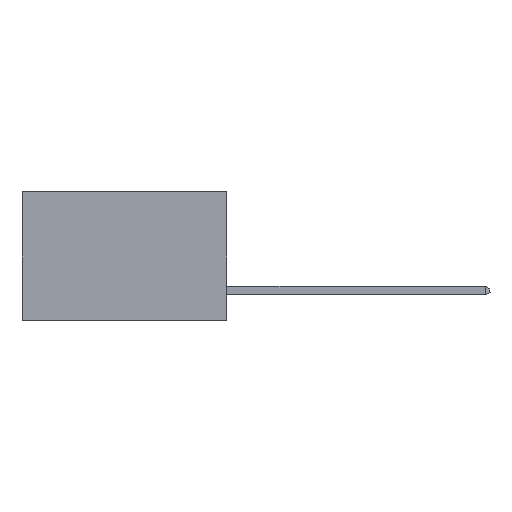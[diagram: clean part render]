
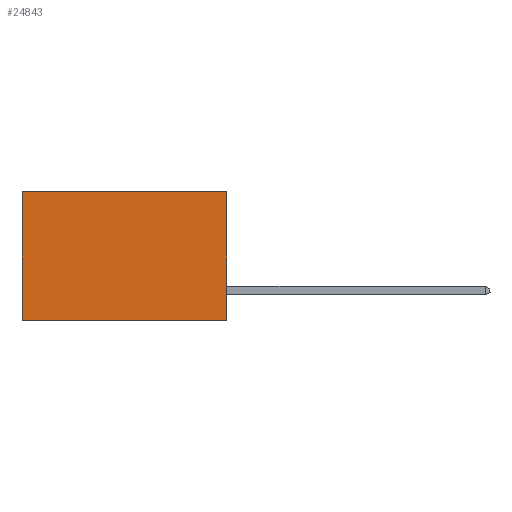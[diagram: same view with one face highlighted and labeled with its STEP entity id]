
A CAD part, left-side view. The second image highlights one B-rep face of the part: STEP entity #24843.
In plain terms, the highlighted planar face has unit normal (-1, 0, 0).
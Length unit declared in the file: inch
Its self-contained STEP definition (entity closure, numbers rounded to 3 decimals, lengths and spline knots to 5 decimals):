
#1145 = CARTESIAN_POINT ( 'NONE',  ( 0.277, 0., -0.37 ) ) ;
#1520 = EDGE_CURVE ( 'NONE', #19059, #19268, #6909, .T. ) ;
#1739 = CARTESIAN_POINT ( 'NONE',  ( 0.277, 0., -0.37 ) ) ;
#2838 = ORIENTED_EDGE ( 'NONE', *, *, #18835, .F. ) ;
#3963 = EDGE_CURVE ( 'NONE', #24043, #19268, #14627, .T. ) ;
#4383 = EDGE_CURVE ( 'NONE', #18365, #24043, #24876, .T. ) ;
#4741 = VECTOR ( 'NONE', #11171, 39.37008 ) ;
#6909 = LINE ( 'NONE', #17982, #11631 ) ;
#7539 = CARTESIAN_POINT ( 'NONE',  ( 0.277, 0., 0. ) ) ;
#7688 = DIRECTION ( 'NONE',  ( 0., 1., 0. ) ) ;
#8595 = PLANE ( 'NONE',  #10168 ) ;
#8858 = ORIENTED_EDGE ( 'NONE', *, *, #4383, .T. ) ;
#9208 = VECTOR ( 'NONE', #7688, 39.37008 ) ;
#10168 = AXIS2_PLACEMENT_3D ( 'NONE', #20492, #10672, #24343 ) ;
#10672 = DIRECTION ( 'NONE',  ( 1., 0., 0. ) ) ;
#11171 = DIRECTION ( 'NONE',  ( 0., 0., -1. ) ) ;
#11631 = VECTOR ( 'NONE', #25083, 39.37008 ) ;
#11786 = EDGE_LOOP ( 'NONE', ( #14855, #16091, #2838, #8858 ) ) ;
#14627 = LINE ( 'NONE', #15504, #24300 ) ;
#14855 = ORIENTED_EDGE ( 'NONE', *, *, #3963, .T. ) ;
#15453 = DIRECTION ( 'NONE',  ( 0., 0., -1. ) ) ;
#15504 = CARTESIAN_POINT ( 'NONE',  ( 0.277, 0.59, -0.37 ) ) ;
#16091 = ORIENTED_EDGE ( 'NONE', *, *, #1520, .F. ) ;
#17982 = CARTESIAN_POINT ( 'NONE',  ( 0.277, 0., -0.37 ) ) ;
#18212 = CARTESIAN_POINT ( 'NONE',  ( 0.277, 0.59, -0.37 ) ) ;
#18365 = VERTEX_POINT ( 'NONE', #19540 ) ;
#18835 = EDGE_CURVE ( 'NONE', #18365, #19059, #20574, .T. ) ;
#19059 = VERTEX_POINT ( 'NONE', #1739 ) ;
#19241 = FACE_OUTER_BOUND ( 'NONE', #11786, .T. ) ;
#19268 = VERTEX_POINT ( 'NONE', #18212 ) ;
#19540 = CARTESIAN_POINT ( 'NONE',  ( 0.277, 0., 0. ) ) ;
#20013 = CARTESIAN_POINT ( 'NONE',  ( 0.277, 0.59, 0. ) ) ;
#20492 = CARTESIAN_POINT ( 'NONE',  ( 0.277, 0., -0.37 ) ) ;
#20574 = LINE ( 'NONE', #1145, #4741 ) ;
#24043 = VERTEX_POINT ( 'NONE', #20013 ) ;
#24300 = VECTOR ( 'NONE', #15453, 39.37008 ) ;
#24343 = DIRECTION ( 'NONE',  ( 0., 0., -1. ) ) ;
#24843 = ADVANCED_FACE ( 'NONE', ( #19241 ), #8595, .F. ) ;
#24876 = LINE ( 'NONE', #7539, #9208 ) ;
#25083 = DIRECTION ( 'NONE',  ( 0., 1., 0. ) ) ;
